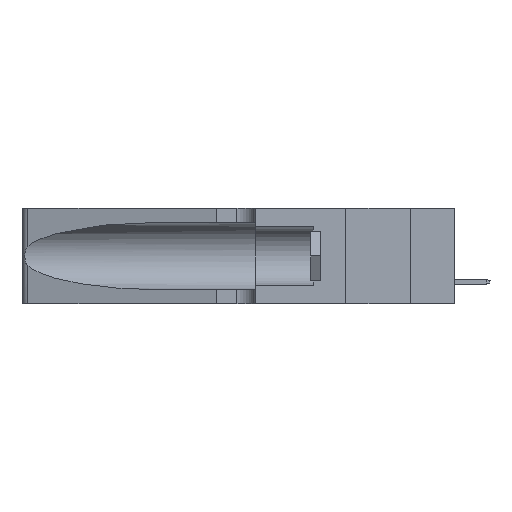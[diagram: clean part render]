
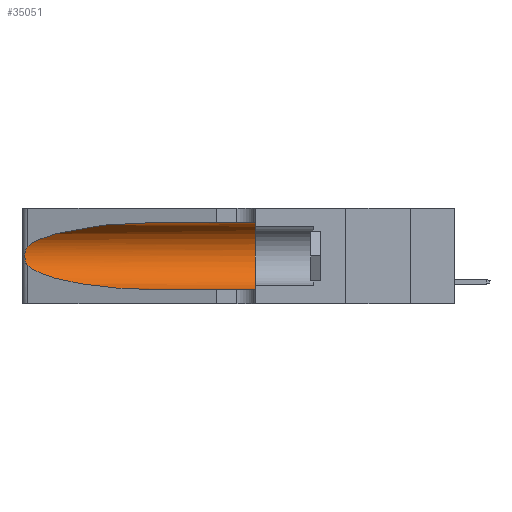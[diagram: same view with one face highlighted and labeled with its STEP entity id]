
A CAD part, left-side view. The second image highlights one B-rep face of the part: STEP entity #35051.
In plain terms, the highlighted cylindrical face has radius 3.308 mm (diameter 6.617 mm), a partial arc.
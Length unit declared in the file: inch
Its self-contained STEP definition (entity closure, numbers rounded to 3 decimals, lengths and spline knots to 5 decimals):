
#1862 = EDGE_CURVE ( 'NONE', #2808, #16968, #21138, .T. ) ;
#2498 = ORIENTED_EDGE ( 'NONE', *, *, #9741, .F. ) ;
#2808 = VERTEX_POINT ( 'NONE', #17731 ) ;
#3204 = CARTESIAN_POINT ( 'NONE',  ( 0.2373, 1.15595, 0.08982 ) ) ;
#4633 = CARTESIAN_POINT ( 'NONE',  ( 0.25487, 1.22718, 0.22369 ) ) ;
#4865 = CARTESIAN_POINT ( 'NONE',  ( 0.26017, 1.23833, 0.17102 ) ) ;
#5318 = CARTESIAN_POINT ( 'NONE',  ( 0.25639, 1.23184, 0.21858 ) ) ;
#6446 = ORIENTED_EDGE ( 'NONE', *, *, #17260, .T. ) ;
#6466 = DIRECTION ( 'NONE',  ( 0., -1., 0. ) ) ;
#6884 = CARTESIAN_POINT ( 'NONE',  ( 0.1305, 1.61858, 0.05475 ) ) ;
#8337 = CARTESIAN_POINT ( 'NONE',  ( 0.25555, 1.22993, 0.14849 ) ) ;
#8602 = CARTESIAN_POINT ( 'NONE',  ( 0.1305, 1.61858, 0.31525 ) ) ;
#9467 = CYLINDRICAL_SURFACE ( 'NONE', #37809, 0.13025 ) ;
#9741 = EDGE_CURVE ( 'NONE', #11607, #24412, #21389, .T. ) ;
#10280 = CARTESIAN_POINT ( 'NONE',  ( 0.1305, 0.72297, 0.31525 ) ) ;
#10361 = CARTESIAN_POINT ( 'NONE',  ( 0.1305, 0.72297, 0.05475 ) ) ;
#11301 = VECTOR ( 'NONE', #32672, 39.37008 ) ;
#11435 = VECTOR ( 'NONE', #28394, 39.37008 ) ;
#11607 = VERTEX_POINT ( 'NONE', #32714 ) ;
#11870 = CARTESIAN_POINT ( 'NONE',  ( 0.1305, 0.72297, 0.05475 ) ) ;
#12482 = CARTESIAN_POINT ( 'NONE',  ( 0.1305, 1.61858, 0.185 ) ) ;
#13281 = EDGE_CURVE ( 'NONE', #32643, #11607, #33135, .T. ) ;
#13533 = CARTESIAN_POINT ( 'NONE',  ( 0.18966, 0.96281, 0.31525 ) ) ;
#14269 = LINE ( 'NONE', #6884, #11435 ) ;
#14810 = VERTEX_POINT ( 'NONE', #11870 ) ;
#15288 = CARTESIAN_POINT ( 'NONE',  ( 0.25789, 1.23486, 0.15765 ) ) ;
#16370 = CARTESIAN_POINT ( 'NONE',  ( 0.25487, 1.22718, 0.14631 ) ) ;
#16968 = VERTEX_POINT ( 'NONE', #16370 ) ;
#17260 = EDGE_CURVE ( 'NONE', #14810, #24412, #14269, .T. ) ;
#17307 = CARTESIAN_POINT ( 'NONE',  ( 0.18966, 0.96281, 0.05475 ) ) ;
#17633 = DIRECTION ( 'NONE',  ( 0., 0., 1. ) ) ;
#17731 = CARTESIAN_POINT ( 'NONE',  ( 0.25487, 1.22718, 0.22369 ) ) ;
#18974 = CARTESIAN_POINT ( 'NONE',  ( 0.25854, 1.2359, 0.20912 ) ) ;
#19427 = CARTESIAN_POINT ( 'NONE',  ( 0.26075, 1.23896, 0.19203 ) ) ;
#19660 = DIRECTION ( 'NONE',  ( 0., 0., -1. ) ) ;
#21138 = B_SPLINE_CURVE_WITH_KNOTS ( 'NONE', 3,
 ( #4633, #36341, #5318, #36575, #18974, #23125, #19427, #40033, #4865, #26391, #15288, #22203, #8337, #30088 ),
 .UNSPECIFIED., .F., .F.,
 ( 4, 2, 2, 2, 2, 2, 4 ),
 ( 0., 0.00027, 0.00053, 0.00107, 0.0016, 0.00187, 0.00214 ),
 .UNSPECIFIED. ) ;
#21389 = CIRCLE ( 'NONE', #31764, 0.13025 ) ;
#22203 = CARTESIAN_POINT ( 'NONE',  ( 0.25639, 1.23186, 0.15144 ) ) ;
#23125 = CARTESIAN_POINT ( 'NONE',  ( 0.26018, 1.23835, 0.19895 ) ) ;
#24412 = VERTEX_POINT ( 'NONE', #32727 ) ;
#26391 = CARTESIAN_POINT ( 'NONE',  ( 0.25856, 1.23593, 0.16098 ) ) ;
#28185 = CARTESIAN_POINT ( 'NONE',  ( 0.1305, 0.72297, 0.31525 ) ) ;
#28332 =( BOUNDED_CURVE ( )  B_SPLINE_CURVE ( 3, ( #10280, #13533, #38757, #42217 ),
 .UNSPECIFIED., .F., .T. ) 
 B_SPLINE_CURVE_WITH_KNOTS ( ( 4, 4 ),
 ( 1.5708, 2.84003 ),
 .UNSPECIFIED. ) 
 CURVE ( )  GEOMETRIC_REPRESENTATION_ITEM ( )  RATIONAL_B_SPLINE_CURVE ( ( 1., 0.87, 0.87, 1. ) ) 
 REPRESENTATION_ITEM ( '' )  );
#28394 = DIRECTION ( 'NONE',  ( 0., -1., 0. ) ) ;
#28529 = DIRECTION ( 'NONE',  ( 0., 1., 0. ) ) ;
#28741 = CARTESIAN_POINT ( 'NONE',  ( 0.1305, 0.35, 0.185 ) ) ;
#29146 = EDGE_CURVE ( 'NONE', #32643, #2808, #28332, .T. ) ;
#30088 = CARTESIAN_POINT ( 'NONE',  ( 0.25487, 1.22718, 0.14631 ) ) ;
#31291 =( BOUNDED_CURVE ( )  B_SPLINE_CURVE ( 3, ( #34895, #3204, #17307, #10361 ),
 .UNSPECIFIED., .F., .T. ) 
 B_SPLINE_CURVE_WITH_KNOTS ( ( 4, 4 ),
 ( 3.44316, 4.71239 ),
 .UNSPECIFIED. ) 
 CURVE ( )  GEOMETRIC_REPRESENTATION_ITEM ( )  RATIONAL_B_SPLINE_CURVE ( ( 1., 0.87, 0.87, 1. ) ) 
 REPRESENTATION_ITEM ( '' )  );
#31764 = AXIS2_PLACEMENT_3D ( 'NONE', #28741, #28529, #17633 ) ;
#32632 = EDGE_CURVE ( 'NONE', #16968, #14810, #31291, .T. ) ;
#32643 = VERTEX_POINT ( 'NONE', #28185 ) ;
#32672 = DIRECTION ( 'NONE',  ( 0., -1., 0. ) ) ;
#32714 = CARTESIAN_POINT ( 'NONE',  ( 0.1305, 0.35, 0.31525 ) ) ;
#32727 = CARTESIAN_POINT ( 'NONE',  ( 0.1305, 0.35, 0.05475 ) ) ;
#33135 = LINE ( 'NONE', #8602, #11301 ) ;
#33723 = EDGE_LOOP ( 'NONE', ( #41593, #42258, #38644, #6446, #2498, #42644 ) ) ;
#34895 = CARTESIAN_POINT ( 'NONE',  ( 0.25487, 1.22718, 0.14631 ) ) ;
#35051 = ADVANCED_FACE ( 'NONE', ( #41181 ), #9467, .F. ) ;
#36341 = CARTESIAN_POINT ( 'NONE',  ( 0.25555, 1.22994, 0.2215 ) ) ;
#36575 = CARTESIAN_POINT ( 'NONE',  ( 0.25787, 1.23484, 0.2124 ) ) ;
#37809 = AXIS2_PLACEMENT_3D ( 'NONE', #12482, #6466, #19660 ) ;
#38644 = ORIENTED_EDGE ( 'NONE', *, *, #32632, .T. ) ;
#38757 = CARTESIAN_POINT ( 'NONE',  ( 0.2373, 1.15595, 0.28018 ) ) ;
#40033 = CARTESIAN_POINT ( 'NONE',  ( 0.26075, 1.23896, 0.178 ) ) ;
#41181 = FACE_OUTER_BOUND ( 'NONE', #33723, .T. ) ;
#41593 = ORIENTED_EDGE ( 'NONE', *, *, #29146, .T. ) ;
#42217 = CARTESIAN_POINT ( 'NONE',  ( 0.25487, 1.22718, 0.22369 ) ) ;
#42258 = ORIENTED_EDGE ( 'NONE', *, *, #1862, .T. ) ;
#42644 = ORIENTED_EDGE ( 'NONE', *, *, #13281, .F. ) ;
